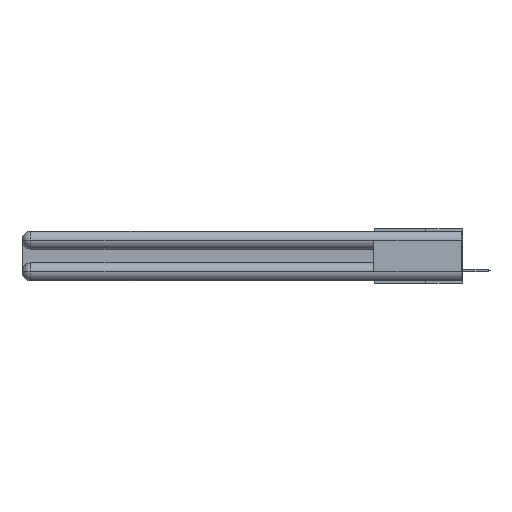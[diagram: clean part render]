
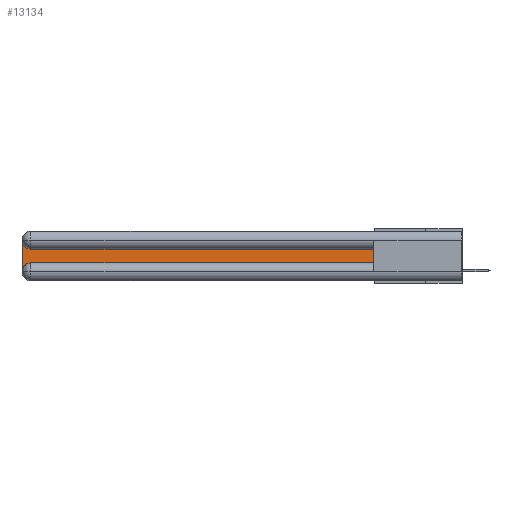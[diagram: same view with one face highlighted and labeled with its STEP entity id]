
A CAD part, left-side view. The second image highlights one B-rep face of the part: STEP entity #13134.
In plain terms, the highlighted planar face has unit normal (-1, 0, 0).
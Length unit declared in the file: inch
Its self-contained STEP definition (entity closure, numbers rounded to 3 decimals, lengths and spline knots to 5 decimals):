
#1504 = ORIENTED_EDGE ( 'NONE', *, *, #16239, .T. ) ;
#1640 = CARTESIAN_POINT ( 'NONE',  ( 0.075, 2.94, -0.2775 ) ) ;
#1733 = DIRECTION ( 'NONE',  ( 1., 0., 0. ) ) ;
#1827 = ORIENTED_EDGE ( 'NONE', *, *, #15565, .T. ) ;
#4043 = DIRECTION ( 'NONE',  ( 1., 0., 0. ) ) ;
#4125 = CARTESIAN_POINT ( 'NONE',  ( 0.075, 3., -0.1225 ) ) ;
#4796 = VERTEX_POINT ( 'NONE', #21042 ) ;
#5311 = FACE_OUTER_BOUND ( 'NONE', #20154, .T. ) ;
#5360 = CARTESIAN_POINT ( 'NONE',  ( 0.075, 2.94, -0.2175 ) ) ;
#5465 = LINE ( 'NONE', #20958, #14044 ) ;
#6915 = CARTESIAN_POINT ( 'NONE',  ( 0.075, 0.6, -0.2175 ) ) ;
#6969 = LINE ( 'NONE', #14502, #8245 ) ;
#6996 = EDGE_CURVE ( 'NONE', #16156, #11982, #14586, .T. ) ;
#7381 = AXIS2_PLACEMENT_3D ( 'NONE', #11002, #23123, #23290 ) ;
#7852 = EDGE_CURVE ( 'NONE', #4796, #23540, #16446, .T. ) ;
#7992 = VERTEX_POINT ( 'NONE', #15493 ) ;
#8245 = VECTOR ( 'NONE', #10188, 39.37008 ) ;
#8624 = DIRECTION ( 'NONE',  ( 0., -1., 0. ) ) ;
#9532 = DIRECTION ( 'NONE',  ( 0., 0., -1. ) ) ;
#10188 = DIRECTION ( 'NONE',  ( 0., 1., 0. ) ) ;
#11002 = CARTESIAN_POINT ( 'NONE',  ( 0.075, 2.94, -0.0625 ) ) ;
#11982 = VERTEX_POINT ( 'NONE', #5360 ) ;
#13134 = ADVANCED_FACE ( 'NONE', ( #5311 ), #24526, .F. ) ;
#13598 = LINE ( 'NONE', #6915, #14858 ) ;
#13835 = ORIENTED_EDGE ( 'NONE', *, *, #23525, .T. ) ;
#14044 = VECTOR ( 'NONE', #8624, 39.37008 ) ;
#14307 = CARTESIAN_POINT ( 'NONE',  ( 0.075, 3., -0.2775 ) ) ;
#14502 = CARTESIAN_POINT ( 'NONE',  ( 0.075, 0.6, -0.1225 ) ) ;
#14586 = CIRCLE ( 'NONE', #17858, 0.06 ) ;
#14858 = VECTOR ( 'NONE', #24503, 39.37008 ) ;
#15313 = VERTEX_POINT ( 'NONE', #20427 ) ;
#15493 = CARTESIAN_POINT ( 'NONE',  ( 0.075, 0.6, -0.2175 ) ) ;
#15565 = EDGE_CURVE ( 'NONE', #11982, #7992, #5465, .T. ) ;
#15578 = ORIENTED_EDGE ( 'NONE', *, *, #6996, .T. ) ;
#16156 = VERTEX_POINT ( 'NONE', #14307 ) ;
#16239 = EDGE_CURVE ( 'NONE', #23540, #16156, #16496, .T. ) ;
#16446 = CIRCLE ( 'NONE', #7381, 0.06 ) ;
#16496 = LINE ( 'NONE', #23201, #22175 ) ;
#17167 = EDGE_CURVE ( 'NONE', #15313, #4796, #6969, .T. ) ;
#17858 = AXIS2_PLACEMENT_3D ( 'NONE', #1640, #1733, #9532 ) ;
#18362 = DIRECTION ( 'NONE',  ( 0., 0., -1. ) ) ;
#19259 = DIRECTION ( 'NONE',  ( 0., 0., -1. ) ) ;
#19644 = ORIENTED_EDGE ( 'NONE', *, *, #17167, .T. ) ;
#19910 = ORIENTED_EDGE ( 'NONE', *, *, #7852, .T. ) ;
#19987 = AXIS2_PLACEMENT_3D ( 'NONE', #4125, #4043, #18362 ) ;
#20154 = EDGE_LOOP ( 'NONE', ( #19644, #19910, #1504, #15578, #1827, #13835 ) ) ;
#20427 = CARTESIAN_POINT ( 'NONE',  ( 0.075, 0.6, -0.1225 ) ) ;
#20649 = CARTESIAN_POINT ( 'NONE',  ( 0.075, 3., -0.0625 ) ) ;
#20958 = CARTESIAN_POINT ( 'NONE',  ( 0.075, 0.6, -0.2175 ) ) ;
#21042 = CARTESIAN_POINT ( 'NONE',  ( 0.075, 2.94, -0.1225 ) ) ;
#22175 = VECTOR ( 'NONE', #19259, 39.37008 ) ;
#23123 = DIRECTION ( 'NONE',  ( 1., 0., 0. ) ) ;
#23201 = CARTESIAN_POINT ( 'NONE',  ( 0.075, 3., -0.2175 ) ) ;
#23290 = DIRECTION ( 'NONE',  ( 0., 0., -1. ) ) ;
#23525 = EDGE_CURVE ( 'NONE', #7992, #15313, #13598, .T. ) ;
#23540 = VERTEX_POINT ( 'NONE', #20649 ) ;
#24503 = DIRECTION ( 'NONE',  ( 0., 0., 1. ) ) ;
#24526 = PLANE ( 'NONE',  #19987 ) ;
